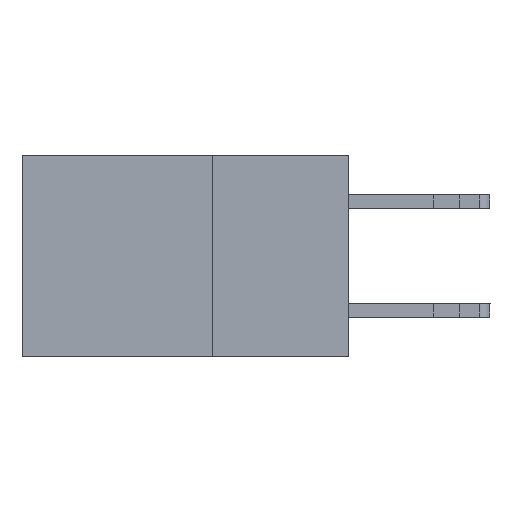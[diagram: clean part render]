
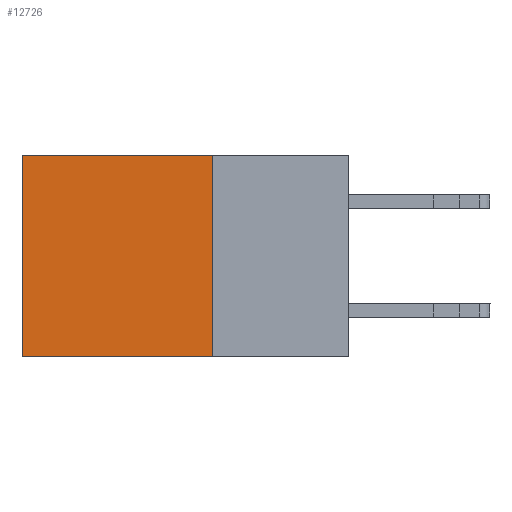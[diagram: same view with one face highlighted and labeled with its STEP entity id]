
A CAD part, left-side view. The second image highlights one B-rep face of the part: STEP entity #12726.
In plain terms, the highlighted planar face has unit normal (-1, 0, 0).
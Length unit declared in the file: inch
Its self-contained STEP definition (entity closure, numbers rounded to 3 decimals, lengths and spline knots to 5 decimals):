
#138 = CARTESIAN_POINT ( 'NONE',  ( 0.298, 0.6, 0. ) ) ;
#413 = CARTESIAN_POINT ( 'NONE',  ( 0.298, 0.25, -0.37 ) ) ;
#678 = EDGE_LOOP ( 'NONE', ( #2009, #1285, #12407, #9636 ) ) ;
#981 = CARTESIAN_POINT ( 'NONE',  ( 0.298, 0.25, 0. ) ) ;
#1285 = ORIENTED_EDGE ( 'NONE', *, *, #4521, .F. ) ;
#1317 = CARTESIAN_POINT ( 'NONE',  ( 0.298, 0.6, -0.37 ) ) ;
#1532 = LINE ( 'NONE', #981, #10173 ) ;
#1754 = CARTESIAN_POINT ( 'NONE',  ( 0.298, 0.25, 0. ) ) ;
#1950 = LINE ( 'NONE', #14578, #4877 ) ;
#2009 = ORIENTED_EDGE ( 'NONE', *, *, #7193, .T. ) ;
#2327 = DIRECTION ( 'NONE',  ( 0., 0., -1. ) ) ;
#2336 = VECTOR ( 'NONE', #10467, 39.37008 ) ;
#2928 = FACE_OUTER_BOUND ( 'NONE', #678, .T. ) ;
#3272 = CARTESIAN_POINT ( 'NONE',  ( 0.298, 0.25, 0. ) ) ;
#4442 = DIRECTION ( 'NONE',  ( 0., 0., -1. ) ) ;
#4521 = EDGE_CURVE ( 'NONE', #4838, #14348, #9400, .T. ) ;
#4838 = VERTEX_POINT ( 'NONE', #15941 ) ;
#4877 = VECTOR ( 'NONE', #4442, 39.37008 ) ;
#5395 = VERTEX_POINT ( 'NONE', #3272 ) ;
#5627 = DIRECTION ( 'NONE',  ( 1., 0., 0. ) ) ;
#7161 = DIRECTION ( 'NONE',  ( 0., 0., -1. ) ) ;
#7193 = EDGE_CURVE ( 'NONE', #13118, #14348, #1950, .T. ) ;
#7581 = LINE ( 'NONE', #8508, #15848 ) ;
#8424 = PLANE ( 'NONE',  #11793 ) ;
#8508 = CARTESIAN_POINT ( 'NONE',  ( 0.298, 0.25, 0. ) ) ;
#8528 = EDGE_CURVE ( 'NONE', #5395, #13118, #1532, .T. ) ;
#9400 = LINE ( 'NONE', #413, #2336 ) ;
#9636 = ORIENTED_EDGE ( 'NONE', *, *, #8528, .T. ) ;
#10173 = VECTOR ( 'NONE', #12313, 39.37008 ) ;
#10467 = DIRECTION ( 'NONE',  ( 0., 1., 0. ) ) ;
#11793 = AXIS2_PLACEMENT_3D ( 'NONE', #1754, #5627, #7161 ) ;
#12313 = DIRECTION ( 'NONE',  ( 0., 1., 0. ) ) ;
#12407 = ORIENTED_EDGE ( 'NONE', *, *, #16050, .F. ) ;
#12726 = ADVANCED_FACE ( 'NONE', ( #2928 ), #8424, .F. ) ;
#13118 = VERTEX_POINT ( 'NONE', #138 ) ;
#14348 = VERTEX_POINT ( 'NONE', #1317 ) ;
#14578 = CARTESIAN_POINT ( 'NONE',  ( 0.298, 0.6, 0. ) ) ;
#15848 = VECTOR ( 'NONE', #2327, 39.37008 ) ;
#15941 = CARTESIAN_POINT ( 'NONE',  ( 0.298, 0.25, -0.37 ) ) ;
#16050 = EDGE_CURVE ( 'NONE', #5395, #4838, #7581, .T. ) ;
